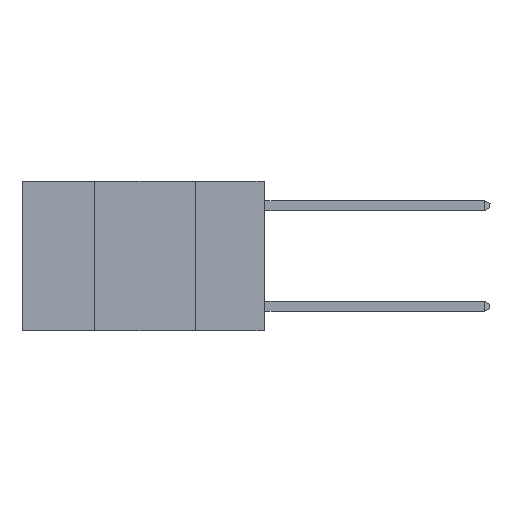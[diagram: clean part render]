
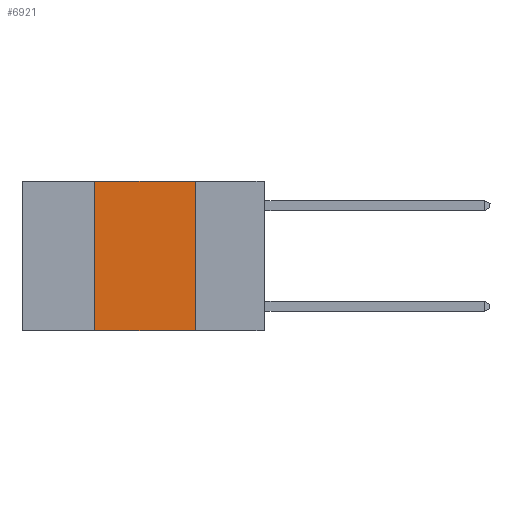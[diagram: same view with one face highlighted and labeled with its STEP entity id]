
A CAD part, left-side view. The second image highlights one B-rep face of the part: STEP entity #6921.
In plain terms, the highlighted planar face has unit normal (-1, 0, 0).
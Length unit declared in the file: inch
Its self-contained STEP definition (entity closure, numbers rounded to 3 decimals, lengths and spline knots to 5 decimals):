
#9 = EDGE_CURVE ( 'NONE', #2767, #14951, #3317, .T. ) ;
#159 = CARTESIAN_POINT ( 'NONE',  ( 0., 0.42, 0. ) ) ;
#784 = VECTOR ( 'NONE', #6359, 39.37008 ) ;
#1194 = EDGE_CURVE ( 'NONE', #19451, #2767, #10903, .T. ) ;
#2262 = DIRECTION ( 'NONE',  ( 0., 0., 1. ) ) ;
#2437 = DIRECTION ( 'NONE',  ( 0., 0., -1. ) ) ;
#2767 = VERTEX_POINT ( 'NONE', #159 ) ;
#3317 = LINE ( 'NONE', #7979, #6183 ) ;
#5579 = LINE ( 'NONE', #10354, #21368 ) ;
#6183 = VECTOR ( 'NONE', #11853, 39.37008 ) ;
#6253 = EDGE_LOOP ( 'NONE', ( #15387, #20501, #8727, #8598 ) ) ;
#6359 = DIRECTION ( 'NONE',  ( 0., -1., 0. ) ) ;
#6921 = ADVANCED_FACE ( 'NONE', ( #15676 ), #8970, .F. ) ;
#7370 = LINE ( 'NONE', #14091, #784 ) ;
#7979 = CARTESIAN_POINT ( 'NONE',  ( 0., 0.6, 0. ) ) ;
#8598 = ORIENTED_EDGE ( 'NONE', *, *, #9344, .T. ) ;
#8727 = ORIENTED_EDGE ( 'NONE', *, *, #1194, .F. ) ;
#8970 = PLANE ( 'NONE',  #11302 ) ;
#9344 = EDGE_CURVE ( 'NONE', #19451, #15326, #7370, .T. ) ;
#10354 = CARTESIAN_POINT ( 'NONE',  ( 0., 0.17, 0. ) ) ;
#10851 = CARTESIAN_POINT ( 'NONE',  ( 0., 0.6, 0. ) ) ;
#10903 = LINE ( 'NONE', #12771, #12417 ) ;
#11302 = AXIS2_PLACEMENT_3D ( 'NONE', #10851, #20753, #2437 ) ;
#11853 = DIRECTION ( 'NONE',  ( 0., -1., 0. ) ) ;
#12417 = VECTOR ( 'NONE', #2262, 39.37008 ) ;
#12429 = CARTESIAN_POINT ( 'NONE',  ( 0., 0.42, -0.37 ) ) ;
#12771 = CARTESIAN_POINT ( 'NONE',  ( 0., 0.42, 0. ) ) ;
#13975 = DIRECTION ( 'NONE',  ( 0., 0., -1. ) ) ;
#14091 = CARTESIAN_POINT ( 'NONE',  ( 0., 0.6, -0.37 ) ) ;
#14951 = VERTEX_POINT ( 'NONE', #19773 ) ;
#15326 = VERTEX_POINT ( 'NONE', #16556 ) ;
#15387 = ORIENTED_EDGE ( 'NONE', *, *, #15915, .F. ) ;
#15676 = FACE_OUTER_BOUND ( 'NONE', #6253, .T. ) ;
#15915 = EDGE_CURVE ( 'NONE', #14951, #15326, #5579, .T. ) ;
#16556 = CARTESIAN_POINT ( 'NONE',  ( 0., 0.17, -0.37 ) ) ;
#19451 = VERTEX_POINT ( 'NONE', #12429 ) ;
#19773 = CARTESIAN_POINT ( 'NONE',  ( 0., 0.17, 0. ) ) ;
#20501 = ORIENTED_EDGE ( 'NONE', *, *, #9, .F. ) ;
#20753 = DIRECTION ( 'NONE',  ( 1., 0., 0. ) ) ;
#21368 = VECTOR ( 'NONE', #13975, 39.37008 ) ;
